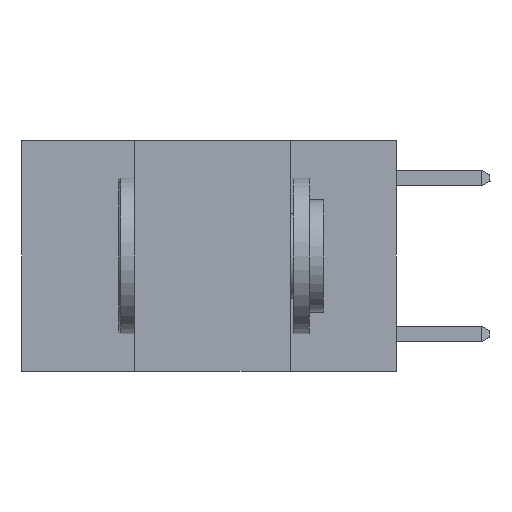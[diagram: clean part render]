
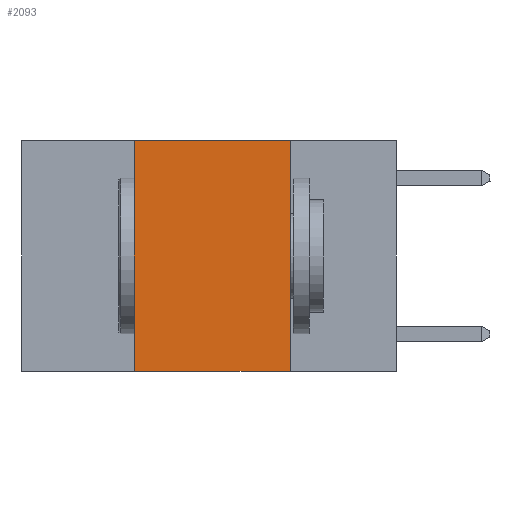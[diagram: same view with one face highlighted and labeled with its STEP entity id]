
A CAD part, left-side view. The second image highlights one B-rep face of the part: STEP entity #2093.
In plain terms, the highlighted planar face has unit normal (-1, 0, 0).
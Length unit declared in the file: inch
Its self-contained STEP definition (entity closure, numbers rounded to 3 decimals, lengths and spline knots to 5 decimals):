
#62 = VERTEX_POINT ( 'NONE', #4748 ) ;
#157 = CARTESIAN_POINT ( 'NONE',  ( 0., 0.17, -0.37 ) ) ;
#294 = DIRECTION ( 'NONE',  ( 0., 0., -1. ) ) ;
#388 = CARTESIAN_POINT ( 'NONE',  ( 0., 0.6, 0. ) ) ;
#517 = ORIENTED_EDGE ( 'NONE', *, *, #7979, .F. ) ;
#1035 = LINE ( 'NONE', #5112, #8999 ) ;
#1075 = DIRECTION ( 'NONE',  ( 0., 0., -1. ) ) ;
#1934 = VECTOR ( 'NONE', #9589, 39.37008 ) ;
#2093 = ADVANCED_FACE ( 'NONE', ( #7421 ), #6023, .F. ) ;
#2145 = CARTESIAN_POINT ( 'NONE',  ( 0., 0.17, 0. ) ) ;
#2284 = ORIENTED_EDGE ( 'NONE', *, *, #7028, .F. ) ;
#2334 = CARTESIAN_POINT ( 'NONE',  ( 0., 0.6, 0. ) ) ;
#2439 = VERTEX_POINT ( 'NONE', #2690 ) ;
#2690 = CARTESIAN_POINT ( 'NONE',  ( 0., 0.42, 0. ) ) ;
#3410 = DIRECTION ( 'NONE',  ( 1., 0., 0. ) ) ;
#3443 = EDGE_LOOP ( 'NONE', ( #517, #7418, #2284, #9266 ) ) ;
#4058 = LINE ( 'NONE', #388, #1934 ) ;
#4748 = CARTESIAN_POINT ( 'NONE',  ( 0., 0.42, -0.37 ) ) ;
#5112 = CARTESIAN_POINT ( 'NONE',  ( 0., 0.17, 0. ) ) ;
#5780 = DIRECTION ( 'NONE',  ( 0., 0., 1. ) ) ;
#6023 = PLANE ( 'NONE',  #8774 ) ;
#6534 = EDGE_CURVE ( 'NONE', #62, #7814, #8668, .T. ) ;
#6718 = CARTESIAN_POINT ( 'NONE',  ( 0., 0.6, -0.37 ) ) ;
#6769 = VECTOR ( 'NONE', #8910, 39.37008 ) ;
#6893 = VECTOR ( 'NONE', #5780, 39.37008 ) ;
#7028 = EDGE_CURVE ( 'NONE', #62, #2439, #9017, .T. ) ;
#7256 = CARTESIAN_POINT ( 'NONE',  ( 0., 0.42, 0. ) ) ;
#7359 = VERTEX_POINT ( 'NONE', #2145 ) ;
#7418 = ORIENTED_EDGE ( 'NONE', *, *, #8676, .F. ) ;
#7421 = FACE_OUTER_BOUND ( 'NONE', #3443, .T. ) ;
#7814 = VERTEX_POINT ( 'NONE', #157 ) ;
#7979 = EDGE_CURVE ( 'NONE', #7359, #7814, #1035, .T. ) ;
#8668 = LINE ( 'NONE', #6718, #6769 ) ;
#8676 = EDGE_CURVE ( 'NONE', #2439, #7359, #4058, .T. ) ;
#8774 = AXIS2_PLACEMENT_3D ( 'NONE', #2334, #3410, #1075 ) ;
#8910 = DIRECTION ( 'NONE',  ( 0., -1., 0. ) ) ;
#8999 = VECTOR ( 'NONE', #294, 39.37008 ) ;
#9017 = LINE ( 'NONE', #7256, #6893 ) ;
#9266 = ORIENTED_EDGE ( 'NONE', *, *, #6534, .T. ) ;
#9589 = DIRECTION ( 'NONE',  ( 0., -1., 0. ) ) ;
